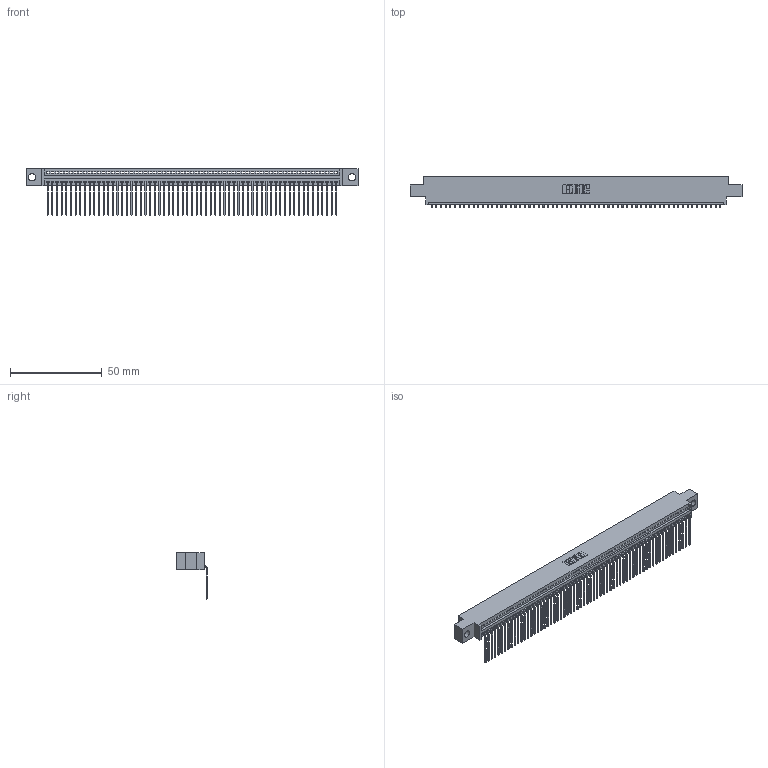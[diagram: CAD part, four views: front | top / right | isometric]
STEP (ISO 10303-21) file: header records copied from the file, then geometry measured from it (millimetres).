
FILE_DESCRIPTION (( 'STEP AP203' ), '1' );
FILE_NAME ('345-063-559-604.STEP', '2019-10-11T12:45:27', ( '' ), ( '' ), 'SwSTEP 2.0', 'SolidWorks 2016', '' );
FILE_SCHEMA (( 'CONFIG_CONTROL_DESIGN' ));
Length unit declared in the file: inch
Products named in the file (3): 345 Part_0.170 Offset - 0.156 Dia-TH; 345-292-001_558 559 Tail - 1; 345-063-559-604
Assembly tree (64 placements, depth 2):
  345-063-559-604
    345 Part_0.170 Offset - 0.156 Dia-TH
    345-292-001_558 559 Tail - 1  x63
Bounding box: 181.23 x 16.75 x 25.53 mm (x, y, z)
Volume: 17394 mm3; surface area: 24569.2 mm2
Topology: 64 solids, 64 shells, 3910 faces, 11819 edges, 7794 vertices
Faces by surface type: plane 2730, cylinder 1180
Entity records: 44807 total; most frequent: CARTESIAN_POINT 7769, ORIENTED_EDGE 7766, DIRECTION 6753, EDGE_CURVE 3883, VECTOR 3499, LINE 3499, VERTEX_POINT 2586, AXIS2_PLACEMENT_3D 1627
